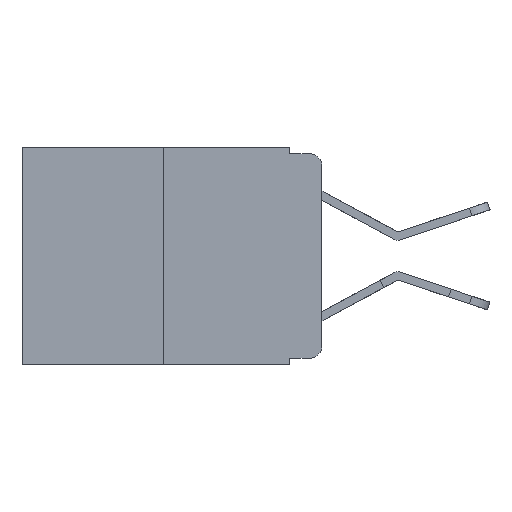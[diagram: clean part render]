
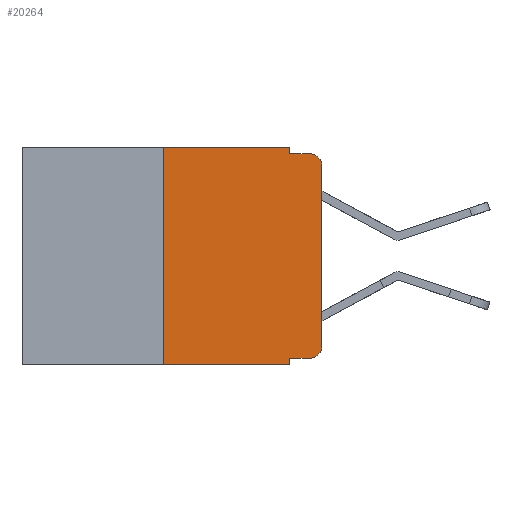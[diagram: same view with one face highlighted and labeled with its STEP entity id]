
A CAD part, left-side view. The second image highlights one B-rep face of the part: STEP entity #20264.
In plain terms, the highlighted planar face has unit normal (-1, 0, 0).
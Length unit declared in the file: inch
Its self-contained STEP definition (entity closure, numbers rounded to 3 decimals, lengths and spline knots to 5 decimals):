
#593 = VECTOR ( 'NONE', #5680, 39.37008 ) ;
#836 = CARTESIAN_POINT ( 'NONE',  ( 0., 0.051, -0.01 ) ) ;
#1799 = CARTESIAN_POINT ( 'NONE',  ( 0., 0.051, 0. ) ) ;
#1803 = CARTESIAN_POINT ( 'NONE',  ( 0., 0.473, 0. ) ) ;
#1875 = EDGE_CURVE ( 'NONE', #23353, #3703, #25577, .T. ) ;
#1967 = AXIS2_PLACEMENT_3D ( 'NONE', #25310, #6838, #23293 ) ;
#2468 = VERTEX_POINT ( 'NONE', #26356 ) ;
#2488 = VECTOR ( 'NONE', #22487, 39.37008 ) ;
#2771 = DIRECTION ( 'NONE',  ( 0., 0., -1. ) ) ;
#3103 = CARTESIAN_POINT ( 'NONE',  ( 0., 0.25, -0.343 ) ) ;
#3140 = CARTESIAN_POINT ( 'NONE',  ( 0., 0.051, -0.343 ) ) ;
#3357 = VECTOR ( 'NONE', #2771, 39.37008 ) ;
#3455 = CARTESIAN_POINT ( 'NONE',  ( 0., 0.051, -0.01 ) ) ;
#3679 = CARTESIAN_POINT ( 'NONE',  ( 0., 0.02, -0.01 ) ) ;
#3703 = VERTEX_POINT ( 'NONE', #836 ) ;
#3774 = DIRECTION ( 'NONE',  ( 0., 0., 1. ) ) ;
#4491 = VECTOR ( 'NONE', #3774, 39.37008 ) ;
#5680 = DIRECTION ( 'NONE',  ( 0., -1., 0. ) ) ;
#5928 = ORIENTED_EDGE ( 'NONE', *, *, #7886, .F. ) ;
#6056 = VERTEX_POINT ( 'NONE', #6357 ) ;
#6357 = CARTESIAN_POINT ( 'NONE',  ( 0., 0.02, -0.333 ) ) ;
#6838 = DIRECTION ( 'NONE',  ( -1., 0., 0. ) ) ;
#7522 = ORIENTED_EDGE ( 'NONE', *, *, #20107, .F. ) ;
#7886 = EDGE_CURVE ( 'NONE', #22154, #25933, #15720, .T. ) ;
#8491 = LINE ( 'NONE', #23056, #26660 ) ;
#8743 = CARTESIAN_POINT ( 'NONE',  ( 0., 0.051, 0. ) ) ;
#8805 = ORIENTED_EDGE ( 'NONE', *, *, #20745, .T. ) ;
#8935 = CIRCLE ( 'NONE', #20657, 0.02 ) ;
#9443 = DIRECTION ( 'NONE',  ( 0., 0., 1. ) ) ;
#9896 = EDGE_CURVE ( 'NONE', #2468, #6056, #16031, .T. ) ;
#10253 = CARTESIAN_POINT ( 'NONE',  ( 0., 0., 0. ) ) ;
#11317 = DIRECTION ( 'NONE',  ( 0., -1., 0. ) ) ;
#11465 = EDGE_LOOP ( 'NONE', ( #20962, #13276, #7522, #17603, #25433, #5928, #17164, #21390, #18612, #8805 ) ) ;
#11758 = CARTESIAN_POINT ( 'NONE',  ( 0., 0.25, 0. ) ) ;
#12127 = VERTEX_POINT ( 'NONE', #26535 ) ;
#12150 = LINE ( 'NONE', #18292, #2488 ) ;
#12333 = DIRECTION ( 'NONE',  ( -1., 0., 0. ) ) ;
#13276 = ORIENTED_EDGE ( 'NONE', *, *, #19954, .T. ) ;
#13759 = LINE ( 'NONE', #17593, #21345 ) ;
#14754 = EDGE_CURVE ( 'NONE', #22154, #23676, #13759, .T. ) ;
#14974 = VECTOR ( 'NONE', #9443, 39.37008 ) ;
#15068 = CARTESIAN_POINT ( 'NONE',  ( 0., 0.02, -0.313 ) ) ;
#15170 = DIRECTION ( 'NONE',  ( 0., -1., 0. ) ) ;
#15720 = LINE ( 'NONE', #11758, #14974 ) ;
#15946 = FACE_OUTER_BOUND ( 'NONE', #11465, .T. ) ;
#16031 = LINE ( 'NONE', #24311, #593 ) ;
#17164 = ORIENTED_EDGE ( 'NONE', *, *, #14754, .T. ) ;
#17593 = CARTESIAN_POINT ( 'NONE',  ( 0., 0.473, -0.343 ) ) ;
#17603 = ORIENTED_EDGE ( 'NONE', *, *, #1875, .F. ) ;
#18169 = EDGE_CURVE ( 'NONE', #12127, #20152, #22364, .T. ) ;
#18292 = CARTESIAN_POINT ( 'NONE',  ( 0., 0.051, 0. ) ) ;
#18612 = ORIENTED_EDGE ( 'NONE', *, *, #9896, .T. ) ;
#19337 = VECTOR ( 'NONE', #19490, 39.37008 ) ;
#19490 = DIRECTION ( 'NONE',  ( 0., -1., 0. ) ) ;
#19555 = EDGE_CURVE ( 'NONE', #25933, #23353, #8491, .T. ) ;
#19954 = EDGE_CURVE ( 'NONE', #20152, #23857, #20618, .T. ) ;
#20036 = CARTESIAN_POINT ( 'NONE',  ( 0., 0., -0.03 ) ) ;
#20107 = EDGE_CURVE ( 'NONE', #3703, #23857, #22050, .T. ) ;
#20152 = VERTEX_POINT ( 'NONE', #20036 ) ;
#20264 = ADVANCED_FACE ( 'NONE', ( #15946 ), #20427, .F. ) ;
#20427 = PLANE ( 'NONE',  #26694 ) ;
#20618 = CIRCLE ( 'NONE', #1967, 0.02 ) ;
#20657 = AXIS2_PLACEMENT_3D ( 'NONE', #15068, #12333, #23225 ) ;
#20745 = EDGE_CURVE ( 'NONE', #6056, #12127, #8935, .T. ) ;
#20962 = ORIENTED_EDGE ( 'NONE', *, *, #18169, .T. ) ;
#21345 = VECTOR ( 'NONE', #11317, 39.37008 ) ;
#21390 = ORIENTED_EDGE ( 'NONE', *, *, #26167, .F. ) ;
#22050 = LINE ( 'NONE', #3455, #19337 ) ;
#22154 = VERTEX_POINT ( 'NONE', #3103 ) ;
#22364 = LINE ( 'NONE', #10253, #4491 ) ;
#22487 = DIRECTION ( 'NONE',  ( 0., 0., -1. ) ) ;
#22707 = DIRECTION ( 'NONE',  ( 0., 0., -1. ) ) ;
#23056 = CARTESIAN_POINT ( 'NONE',  ( 0., 0.473, 0. ) ) ;
#23225 = DIRECTION ( 'NONE',  ( 0., 0., -1. ) ) ;
#23293 = DIRECTION ( 'NONE',  ( 0., 0., -1. ) ) ;
#23353 = VERTEX_POINT ( 'NONE', #1799 ) ;
#23676 = VERTEX_POINT ( 'NONE', #3140 ) ;
#23857 = VERTEX_POINT ( 'NONE', #3679 ) ;
#24230 = DIRECTION ( 'NONE',  ( 1., 0., 0. ) ) ;
#24311 = CARTESIAN_POINT ( 'NONE',  ( 0., 0.051, -0.333 ) ) ;
#25310 = CARTESIAN_POINT ( 'NONE',  ( 0., 0.02, -0.03 ) ) ;
#25433 = ORIENTED_EDGE ( 'NONE', *, *, #19555, .F. ) ;
#25577 = LINE ( 'NONE', #8743, #3357 ) ;
#25616 = CARTESIAN_POINT ( 'NONE',  ( 0., 0.25, 0. ) ) ;
#25933 = VERTEX_POINT ( 'NONE', #25616 ) ;
#26167 = EDGE_CURVE ( 'NONE', #2468, #23676, #12150, .T. ) ;
#26356 = CARTESIAN_POINT ( 'NONE',  ( 0., 0.051, -0.333 ) ) ;
#26535 = CARTESIAN_POINT ( 'NONE',  ( 0., 0., -0.313 ) ) ;
#26660 = VECTOR ( 'NONE', #15170, 39.37008 ) ;
#26694 = AXIS2_PLACEMENT_3D ( 'NONE', #1803, #24230, #22707 ) ;
